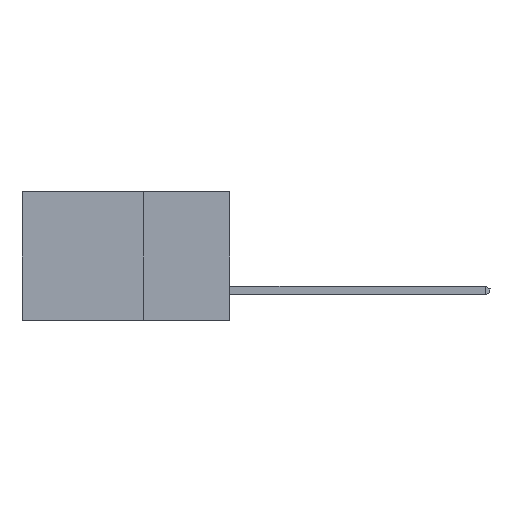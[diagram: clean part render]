
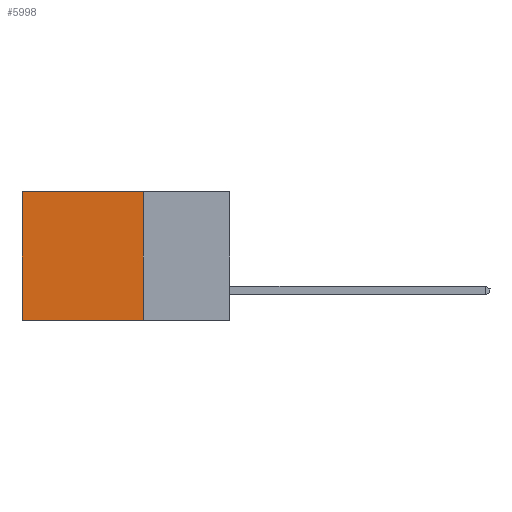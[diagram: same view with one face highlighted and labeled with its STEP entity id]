
A CAD part, left-side view. The second image highlights one B-rep face of the part: STEP entity #5998.
In plain terms, the highlighted planar face has unit normal (-1, 0, 0).
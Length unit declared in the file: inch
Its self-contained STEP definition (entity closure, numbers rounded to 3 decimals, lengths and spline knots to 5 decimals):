
#135 = VECTOR ( 'NONE', #8677, 39.37008 ) ;
#196 = DIRECTION ( 'NONE',  ( 0., 0., -1. ) ) ;
#276 = DIRECTION ( 'NONE',  ( 1., 0., 0. ) ) ;
#617 = DIRECTION ( 'NONE',  ( 0., 1., 0. ) ) ;
#1201 = VERTEX_POINT ( 'NONE', #8066 ) ;
#2024 = EDGE_LOOP ( 'NONE', ( #7376, #7437, #9352, #6450 ) ) ;
#2169 = CARTESIAN_POINT ( 'NONE',  ( 0.2615, 0.6, -0.37 ) ) ;
#2430 = CARTESIAN_POINT ( 'NONE',  ( 0.2615, 0.6, 0. ) ) ;
#2451 = LINE ( 'NONE', #7552, #2718 ) ;
#2718 = VECTOR ( 'NONE', #196, 39.37008 ) ;
#2854 = AXIS2_PLACEMENT_3D ( 'NONE', #6878, #276, #3556 ) ;
#3556 = DIRECTION ( 'NONE',  ( 0., 0., -1. ) ) ;
#3587 = LINE ( 'NONE', #6848, #3657 ) ;
#3617 = FACE_OUTER_BOUND ( 'NONE', #2024, .T. ) ;
#3657 = VECTOR ( 'NONE', #617, 39.37008 ) ;
#4612 = DIRECTION ( 'NONE',  ( 0., 1., 0. ) ) ;
#4662 = CARTESIAN_POINT ( 'NONE',  ( 0.2615, 0.25, -0.37 ) ) ;
#5100 = VERTEX_POINT ( 'NONE', #2430 ) ;
#5323 = EDGE_CURVE ( 'NONE', #9628, #9740, #5407, .T. ) ;
#5387 = LINE ( 'NONE', #6246, #135 ) ;
#5407 = LINE ( 'NONE', #4662, #6164 ) ;
#5998 = ADVANCED_FACE ( 'NONE', ( #3617 ), #7639, .F. ) ;
#6164 = VECTOR ( 'NONE', #4612, 39.37008 ) ;
#6246 = CARTESIAN_POINT ( 'NONE',  ( 0.2615, 0.25, -0.37 ) ) ;
#6450 = ORIENTED_EDGE ( 'NONE', *, *, #6820, .T. ) ;
#6820 = EDGE_CURVE ( 'NONE', #1201, #5100, #3587, .T. ) ;
#6848 = CARTESIAN_POINT ( 'NONE',  ( 0.2615, 0.25, 0. ) ) ;
#6878 = CARTESIAN_POINT ( 'NONE',  ( 0.2615, 0.25, -0.37 ) ) ;
#7376 = ORIENTED_EDGE ( 'NONE', *, *, #8386, .T. ) ;
#7436 = EDGE_CURVE ( 'NONE', #1201, #9628, #5387, .T. ) ;
#7437 = ORIENTED_EDGE ( 'NONE', *, *, #5323, .F. ) ;
#7552 = CARTESIAN_POINT ( 'NONE',  ( 0.2615, 0.6, -0.37 ) ) ;
#7556 = CARTESIAN_POINT ( 'NONE',  ( 0.2615, 0.25, -0.37 ) ) ;
#7639 = PLANE ( 'NONE',  #2854 ) ;
#8066 = CARTESIAN_POINT ( 'NONE',  ( 0.2615, 0.25, 0. ) ) ;
#8386 = EDGE_CURVE ( 'NONE', #5100, #9740, #2451, .T. ) ;
#8677 = DIRECTION ( 'NONE',  ( 0., 0., -1. ) ) ;
#9352 = ORIENTED_EDGE ( 'NONE', *, *, #7436, .F. ) ;
#9628 = VERTEX_POINT ( 'NONE', #7556 ) ;
#9740 = VERTEX_POINT ( 'NONE', #2169 ) ;
